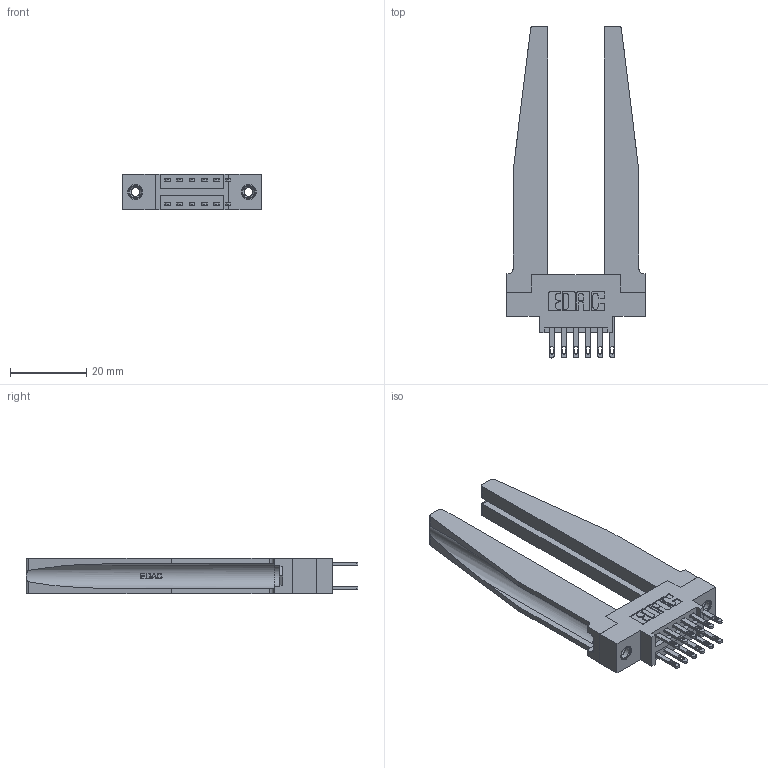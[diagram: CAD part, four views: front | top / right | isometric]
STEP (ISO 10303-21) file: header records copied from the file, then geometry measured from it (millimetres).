
FILE_DESCRIPTION (( 'STEP AP203' ), '1' );
FILE_NAME ('346-012-500-878.STEP', '2022-05-17T18:58:38', ( '' ), ( '' ), 'SwSTEP 2.0', 'SolidWorks 2020', '' );
FILE_SCHEMA (( 'CONFIG_CONTROL_DESIGN' ));
Length unit declared in the file: inch
Products named in the file (5): 346 Part_0.170 Offset - 0.156 Dia-TH; 345-292-001_345-293-100; 345-250-001_345-250-001-102; 346-012-500-878; 346-220-078_345-220-078
Assembly tree (17 placements, depth 2):
  346-012-500-878
    346 Part_0.170 Offset - 0.156 Dia-TH
    345-292-001_345-293-100  x12
    346-220-078_345-220-078  x2
    345-250-001_345-250-001-102  x2
Bounding box: 36.45 x 87.12 x 9.4 mm (x, y, z)
Volume: 10057.7 mm3; surface area: 10727.8 mm2
Topology: 17 solids, 17 shells, 938 faces, 2707 edges, 1794 vertices
Faces by surface type: plane 574, cylinder 312, bspline 36, cone 12, torus 4
Entity records: 13534 total; most frequent: CARTESIAN_POINT 3215, ORIENTED_EDGE 2034, DIRECTION 1875, EDGE_CURVE 1017, LINE 767, VECTOR 767, VERTEX_POINT 672, AXIS2_PLACEMENT_3D 554
